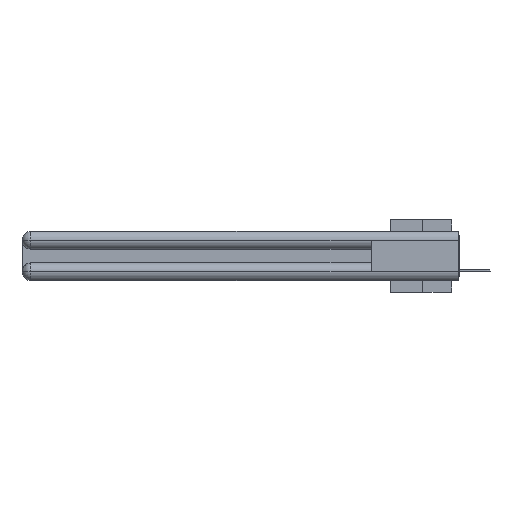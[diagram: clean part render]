
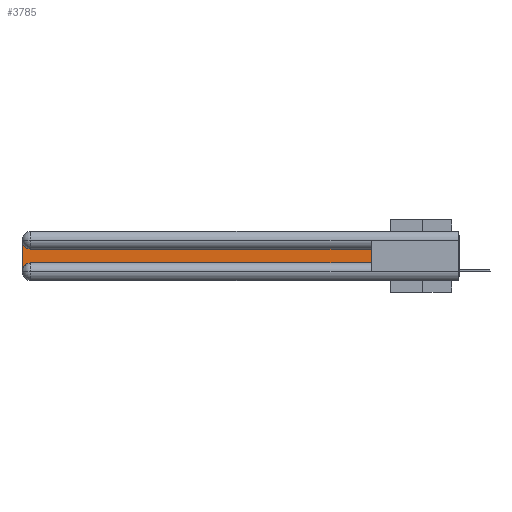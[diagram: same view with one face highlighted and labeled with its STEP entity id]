
A CAD part, left-side view. The second image highlights one B-rep face of the part: STEP entity #3785.
In plain terms, the highlighted planar face has unit normal (-1, 0, 0).
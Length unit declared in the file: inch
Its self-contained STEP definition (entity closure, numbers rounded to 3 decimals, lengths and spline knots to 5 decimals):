
#1132 = DIRECTION ( 'NONE',  ( 1., 0., 0. ) ) ;
#1837 = LINE ( 'NONE', #21402, #4093 ) ;
#3298 = CARTESIAN_POINT ( 'NONE',  ( 0.075, 0.6, -0.2175 ) ) ;
#3785 = ADVANCED_FACE ( 'NONE', ( #28109 ), #8539, .F. ) ;
#3988 = VERTEX_POINT ( 'NONE', #3298 ) ;
#4085 = EDGE_CURVE ( 'NONE', #3988, #15923, #12540, .T. ) ;
#4093 = VECTOR ( 'NONE', #26063, 39.37008 ) ;
#4578 = ORIENTED_EDGE ( 'NONE', *, *, #23431, .T. ) ;
#5893 = ORIENTED_EDGE ( 'NONE', *, *, #24977, .T. ) ;
#6255 = LINE ( 'NONE', #17734, #17123 ) ;
#6883 = ORIENTED_EDGE ( 'NONE', *, *, #12371, .T. ) ;
#7189 = EDGE_LOOP ( 'NONE', ( #4578, #6883, #23759, #12123, #5893, #25964 ) ) ;
#8287 = DIRECTION ( 'NONE',  ( 0., 0., -1. ) ) ;
#8383 = AXIS2_PLACEMENT_3D ( 'NONE', #24895, #10340, #10454 ) ;
#8539 = PLANE ( 'NONE',  #26930 ) ;
#8735 = EDGE_CURVE ( 'NONE', #18124, #14417, #30565, .T. ) ;
#9641 = CARTESIAN_POINT ( 'NONE',  ( 0.075, 2.94, -0.2175 ) ) ;
#10340 = DIRECTION ( 'NONE',  ( 1., 0., 0. ) ) ;
#10454 = DIRECTION ( 'NONE',  ( 0., 0., -1. ) ) ;
#10795 = CARTESIAN_POINT ( 'NONE',  ( 0.075, 3., -0.0625 ) ) ;
#10834 = CARTESIAN_POINT ( 'NONE',  ( 0.075, 2.94, -0.0625 ) ) ;
#11272 = VECTOR ( 'NONE', #31208, 39.37008 ) ;
#12123 = ORIENTED_EDGE ( 'NONE', *, *, #8735, .T. ) ;
#12371 = EDGE_CURVE ( 'NONE', #31173, #25563, #13324, .T. ) ;
#12540 = LINE ( 'NONE', #21845, #23898 ) ;
#13324 = CIRCLE ( 'NONE', #16517, 0.06 ) ;
#13657 = EDGE_CURVE ( 'NONE', #25563, #18124, #1837, .T. ) ;
#14417 = VERTEX_POINT ( 'NONE', #9641 ) ;
#15923 = VERTEX_POINT ( 'NONE', #20765 ) ;
#16517 = AXIS2_PLACEMENT_3D ( 'NONE', #10834, #1132, #8287 ) ;
#16620 = CARTESIAN_POINT ( 'NONE',  ( 0.075, 0.6, -0.1225 ) ) ;
#17123 = VECTOR ( 'NONE', #17631, 39.37008 ) ;
#17631 = DIRECTION ( 'NONE',  ( 0., -1., 0. ) ) ;
#17734 = CARTESIAN_POINT ( 'NONE',  ( 0.075, 0.6, -0.2175 ) ) ;
#18124 = VERTEX_POINT ( 'NONE', #22748 ) ;
#18403 = DIRECTION ( 'NONE',  ( 0., 0., -1. ) ) ;
#20293 = LINE ( 'NONE', #16620, #11272 ) ;
#20765 = CARTESIAN_POINT ( 'NONE',  ( 0.075, 0.6, -0.1225 ) ) ;
#21402 = CARTESIAN_POINT ( 'NONE',  ( 0.075, 3., -0.2175 ) ) ;
#21845 = CARTESIAN_POINT ( 'NONE',  ( 0.075, 0.6, -0.2175 ) ) ;
#22748 = CARTESIAN_POINT ( 'NONE',  ( 0.075, 3., -0.2775 ) ) ;
#23431 = EDGE_CURVE ( 'NONE', #15923, #31173, #20293, .T. ) ;
#23759 = ORIENTED_EDGE ( 'NONE', *, *, #13657, .T. ) ;
#23898 = VECTOR ( 'NONE', #24600, 39.37008 ) ;
#24600 = DIRECTION ( 'NONE',  ( 0., 0., 1. ) ) ;
#24895 = CARTESIAN_POINT ( 'NONE',  ( 0.075, 2.94, -0.2775 ) ) ;
#24977 = EDGE_CURVE ( 'NONE', #14417, #3988, #6255, .T. ) ;
#25404 = CARTESIAN_POINT ( 'NONE',  ( 0.075, 3., -0.1225 ) ) ;
#25563 = VERTEX_POINT ( 'NONE', #10795 ) ;
#25964 = ORIENTED_EDGE ( 'NONE', *, *, #4085, .T. ) ;
#26063 = DIRECTION ( 'NONE',  ( 0., 0., -1. ) ) ;
#26930 = AXIS2_PLACEMENT_3D ( 'NONE', #25404, #30137, #18403 ) ;
#27832 = CARTESIAN_POINT ( 'NONE',  ( 0.075, 2.94, -0.1225 ) ) ;
#28109 = FACE_OUTER_BOUND ( 'NONE', #7189, .T. ) ;
#30137 = DIRECTION ( 'NONE',  ( 1., 0., 0. ) ) ;
#30565 = CIRCLE ( 'NONE', #8383, 0.06 ) ;
#31173 = VERTEX_POINT ( 'NONE', #27832 ) ;
#31208 = DIRECTION ( 'NONE',  ( 0., 1., 0. ) ) ;
